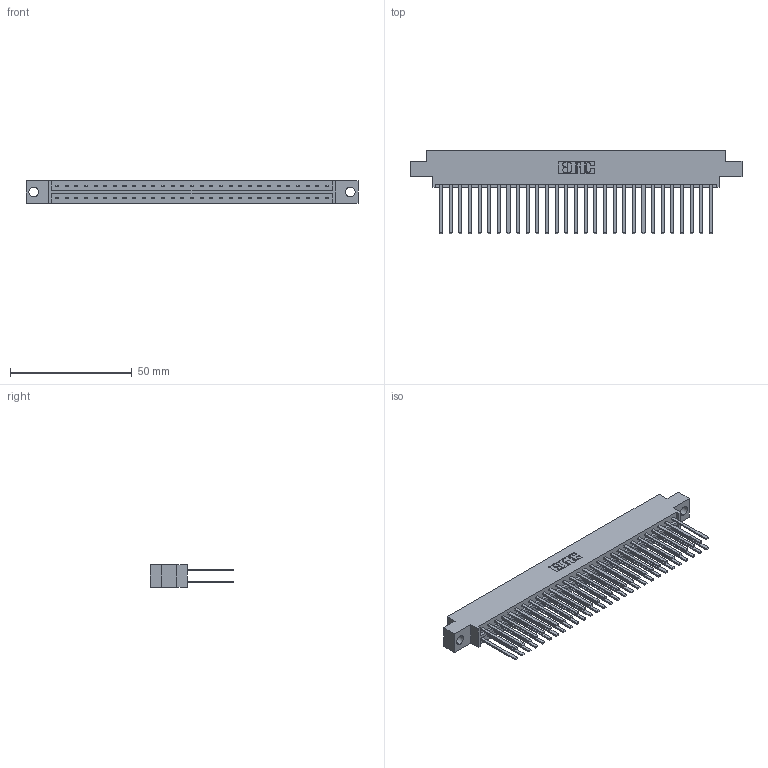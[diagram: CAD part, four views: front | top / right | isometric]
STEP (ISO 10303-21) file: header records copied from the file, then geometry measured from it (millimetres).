
FILE_DESCRIPTION (( 'STEP AP203' ), '1' );
FILE_NAME ('333-058-544-804.STEP', '2018-08-04T06:14:43', ( '' ), ( '' ), 'SwSTEP 2.0', 'SolidWorks 2016', '' );
FILE_SCHEMA (( 'CONFIG_CONTROL_DESIGN' ));
Length unit declared in the file: inch
Products named in the file (3): 333-058-544-804; 333 Part_Offset - .156 Dia - TH; 345-292-001_345-293-144
Assembly tree (59 placements, depth 2):
  333-058-544-804
    333 Part_Offset - .156 Dia - TH
    345-292-001_345-293-144  x58
Bounding box: 136.45 x 34.3 x 9.4 mm (x, y, z)
Volume: 14306.5 mm3; surface area: 19412.2 mm2
Topology: 59 solids, 59 shells, 2786 faces, 8269 edges, 5434 vertices
Faces by surface type: plane 1930, cylinder 856
Entity records: 20289 total; most frequent: CARTESIAN_POINT 3378, ORIENTED_EDGE 3314, DIRECTION 2905, EDGE_CURVE 1657, VECTOR 1533, LINE 1533, VERTEX_POINT 1102, AXIS2_PLACEMENT_3D 686
